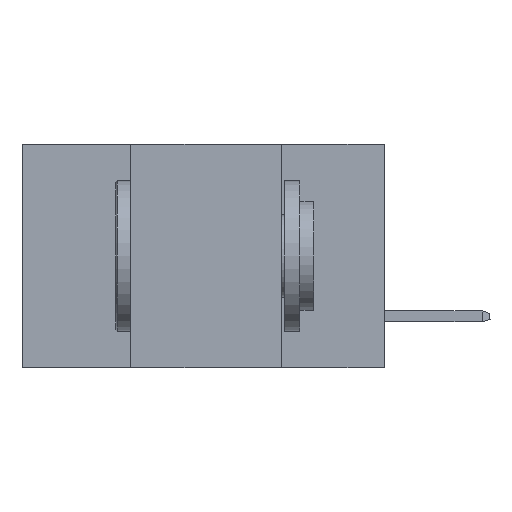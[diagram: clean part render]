
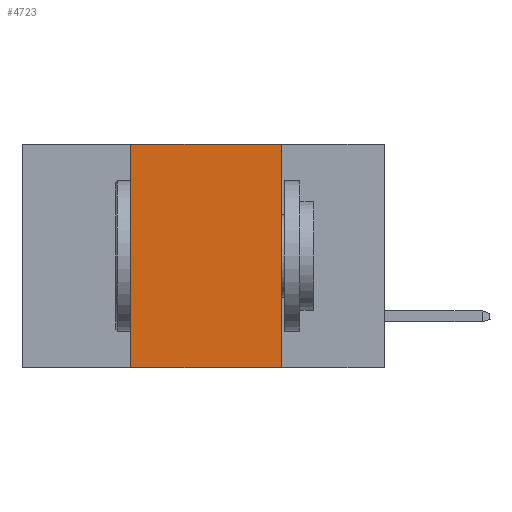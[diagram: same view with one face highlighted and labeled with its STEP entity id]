
A CAD part, left-side view. The second image highlights one B-rep face of the part: STEP entity #4723.
In plain terms, the highlighted planar face has unit normal (-1, 0, 0).
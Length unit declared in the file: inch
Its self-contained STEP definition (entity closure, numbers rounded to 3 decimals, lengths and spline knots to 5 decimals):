
#138 = VERTEX_POINT ( 'NONE', #19504 ) ;
#885 = DIRECTION ( 'NONE',  ( 0., 0., -1. ) ) ;
#895 = DIRECTION ( 'NONE',  ( 0., -1., 0. ) ) ;
#1262 = DIRECTION ( 'NONE',  ( 0., 0., 1. ) ) ;
#1841 = FACE_OUTER_BOUND ( 'NONE', #2424, .T. ) ;
#2080 = ORIENTED_EDGE ( 'NONE', *, *, #7663, .T. ) ;
#2424 = EDGE_LOOP ( 'NONE', ( #21525, #23469, #23001, #2080 ) ) ;
#2581 = LINE ( 'NONE', #7730, #11841 ) ;
#2679 = CARTESIAN_POINT ( 'NONE',  ( 0., 0.17, 0. ) ) ;
#2848 = EDGE_CURVE ( 'NONE', #138, #18717, #21880, .T. ) ;
#4059 = CARTESIAN_POINT ( 'NONE',  ( 0., 0.6, -0.37 ) ) ;
#4723 = ADVANCED_FACE ( 'NONE', ( #1841 ), #23735, .F. ) ;
#6580 = VERTEX_POINT ( 'NONE', #15106 ) ;
#7663 = EDGE_CURVE ( 'NONE', #6580, #14034, #14446, .T. ) ;
#7730 = CARTESIAN_POINT ( 'NONE',  ( 0., 0.17, 0. ) ) ;
#10224 = CARTESIAN_POINT ( 'NONE',  ( 0., 0.6, 0. ) ) ;
#10623 = EDGE_CURVE ( 'NONE', #6580, #138, #22946, .T. ) ;
#10749 = CARTESIAN_POINT ( 'NONE',  ( 0., 0.17, -0.37 ) ) ;
#11558 = DIRECTION ( 'NONE',  ( 0., 0., -1. ) ) ;
#11841 = VECTOR ( 'NONE', #11558, 39.37008 ) ;
#12403 = EDGE_CURVE ( 'NONE', #18717, #14034, #2581, .T. ) ;
#12669 = CARTESIAN_POINT ( 'NONE',  ( 0., 0.42, 0. ) ) ;
#14034 = VERTEX_POINT ( 'NONE', #10749 ) ;
#14446 = LINE ( 'NONE', #4059, #18340 ) ;
#15106 = CARTESIAN_POINT ( 'NONE',  ( 0., 0.42, -0.37 ) ) ;
#16643 = VECTOR ( 'NONE', #1262, 39.37008 ) ;
#18340 = VECTOR ( 'NONE', #19053, 39.37008 ) ;
#18717 = VERTEX_POINT ( 'NONE', #2679 ) ;
#19053 = DIRECTION ( 'NONE',  ( 0., -1., 0. ) ) ;
#19504 = CARTESIAN_POINT ( 'NONE',  ( 0., 0.42, 0. ) ) ;
#19802 = VECTOR ( 'NONE', #895, 39.37008 ) ;
#19970 = CARTESIAN_POINT ( 'NONE',  ( 0., 0.6, 0. ) ) ;
#20489 = AXIS2_PLACEMENT_3D ( 'NONE', #19970, #21884, #885 ) ;
#21525 = ORIENTED_EDGE ( 'NONE', *, *, #12403, .F. ) ;
#21880 = LINE ( 'NONE', #10224, #19802 ) ;
#21884 = DIRECTION ( 'NONE',  ( 1., 0., 0. ) ) ;
#22946 = LINE ( 'NONE', #12669, #16643 ) ;
#23001 = ORIENTED_EDGE ( 'NONE', *, *, #10623, .F. ) ;
#23469 = ORIENTED_EDGE ( 'NONE', *, *, #2848, .F. ) ;
#23735 = PLANE ( 'NONE',  #20489 ) ;
